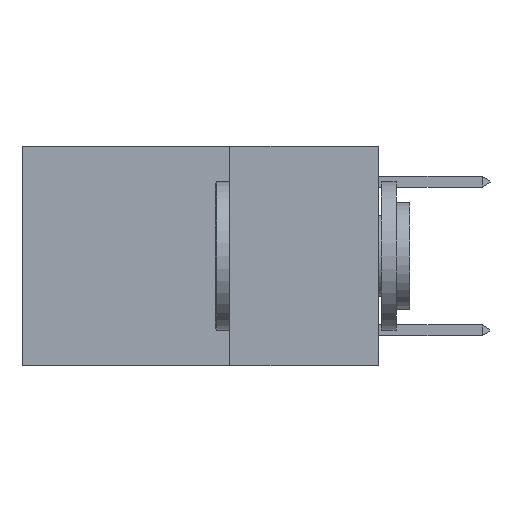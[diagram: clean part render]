
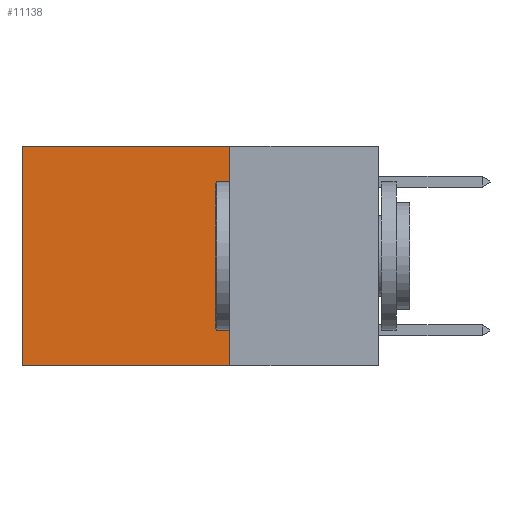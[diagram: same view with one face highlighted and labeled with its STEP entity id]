
A CAD part, left-side view. The second image highlights one B-rep face of the part: STEP entity #11138.
In plain terms, the highlighted planar face has unit normal (-1, 0, 0).
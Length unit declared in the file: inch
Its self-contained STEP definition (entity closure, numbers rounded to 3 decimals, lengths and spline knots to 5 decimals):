
#2019 = EDGE_CURVE ( 'NONE', #6674, #3484, #4919, .T. ) ;
#2045 = CARTESIAN_POINT ( 'NONE',  ( 0.2625, 0.25, 0. ) ) ;
#3170 = VECTOR ( 'NONE', #6562, 39.37008 ) ;
#3475 = DIRECTION ( 'NONE',  ( 0., 0., -1. ) ) ;
#3484 = VERTEX_POINT ( 'NONE', #6174 ) ;
#4919 = LINE ( 'NONE', #14828, #3170 ) ;
#5318 = CARTESIAN_POINT ( 'NONE',  ( 0.2625, 0.25, 0. ) ) ;
#5430 = ORIENTED_EDGE ( 'NONE', *, *, #12753, .F. ) ;
#6174 = CARTESIAN_POINT ( 'NONE',  ( 0.2625, 0.6, -0.37 ) ) ;
#6562 = DIRECTION ( 'NONE',  ( 0., 0., -1. ) ) ;
#6674 = VERTEX_POINT ( 'NONE', #11122 ) ;
#6948 = VECTOR ( 'NONE', #16996, 39.37008 ) ;
#7072 = VECTOR ( 'NONE', #7462, 39.37008 ) ;
#7462 = DIRECTION ( 'NONE',  ( 0., 0., -1. ) ) ;
#8326 = VERTEX_POINT ( 'NONE', #12647 ) ;
#8652 = ORIENTED_EDGE ( 'NONE', *, *, #20341, .T. ) ;
#8657 = VERTEX_POINT ( 'NONE', #17536 ) ;
#11122 = CARTESIAN_POINT ( 'NONE',  ( 0.2625, 0.6, 0. ) ) ;
#11138 = ADVANCED_FACE ( 'NONE', ( #14626 ), #20116, .F. ) ;
#11658 = AXIS2_PLACEMENT_3D ( 'NONE', #2045, #16838, #3475 ) ;
#12647 = CARTESIAN_POINT ( 'NONE',  ( 0.2625, 0.25, 0. ) ) ;
#12753 = EDGE_CURVE ( 'NONE', #8326, #8657, #21030, .T. ) ;
#14186 = CARTESIAN_POINT ( 'NONE',  ( 0.2625, 0.25, 0. ) ) ;
#14195 = EDGE_CURVE ( 'NONE', #8657, #3484, #16589, .T. ) ;
#14626 = FACE_OUTER_BOUND ( 'NONE', #21157, .T. ) ;
#14828 = CARTESIAN_POINT ( 'NONE',  ( 0.2625, 0.6, 0. ) ) ;
#15202 = DIRECTION ( 'NONE',  ( 0., 1., 0. ) ) ;
#15782 = ORIENTED_EDGE ( 'NONE', *, *, #2019, .T. ) ;
#16307 = ORIENTED_EDGE ( 'NONE', *, *, #14195, .F. ) ;
#16589 = LINE ( 'NONE', #20298, #6948 ) ;
#16838 = DIRECTION ( 'NONE',  ( 1., 0., 0. ) ) ;
#16996 = DIRECTION ( 'NONE',  ( 0., 1., 0. ) ) ;
#17536 = CARTESIAN_POINT ( 'NONE',  ( 0.2625, 0.25, -0.37 ) ) ;
#17963 = VECTOR ( 'NONE', #15202, 39.37008 ) ;
#18709 = LINE ( 'NONE', #5318, #17963 ) ;
#20116 = PLANE ( 'NONE',  #11658 ) ;
#20298 = CARTESIAN_POINT ( 'NONE',  ( 0.2625, 0.25, -0.37 ) ) ;
#20341 = EDGE_CURVE ( 'NONE', #8326, #6674, #18709, .T. ) ;
#21030 = LINE ( 'NONE', #14186, #7072 ) ;
#21157 = EDGE_LOOP ( 'NONE', ( #15782, #16307, #5430, #8652 ) ) ;
